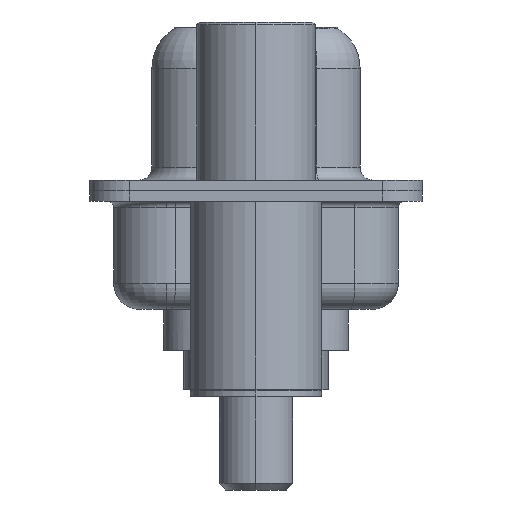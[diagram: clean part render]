
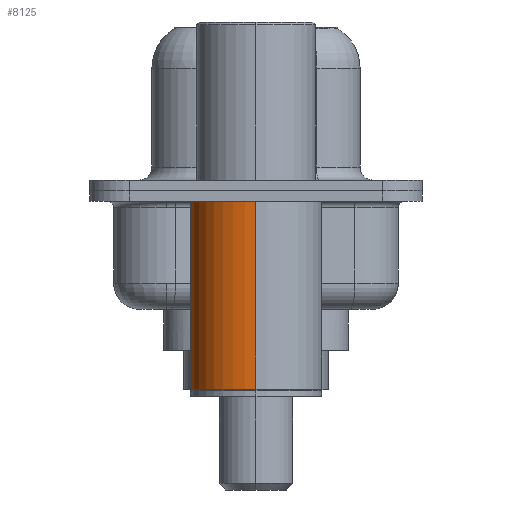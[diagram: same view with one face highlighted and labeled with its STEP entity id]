
A CAD part, left-side view. The second image highlights one B-rep face of the part: STEP entity #8125.
In plain terms, the highlighted cylindrical face has radius 2.5 mm (diameter 5 mm), a partial arc.
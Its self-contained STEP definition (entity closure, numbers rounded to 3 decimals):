
#29 = CARTESIAN_POINT ( 'NONE',  ( 0., 0., 0.581 ) ) ;
#74 = DIRECTION ( 'NONE',  ( 0., 0., 1. ) ) ;
#80 = EDGE_CURVE ( 'NONE', #8897, #9252, #7925, .T. ) ;
#125 = EDGE_CURVE ( 'NONE', #2824, #10675, #13062, .T. ) ;
#345 = AXIS2_PLACEMENT_3D ( 'NONE', #9964, #3302, #11015 ) ;
#373 = AXIS2_PLACEMENT_3D ( 'NONE', #29, #13248, #4343 ) ;
#1049 = VECTOR ( 'NONE', #74, 1000. ) ;
#1395 = CARTESIAN_POINT ( 'NONE',  ( 2.5, 0., 0.581 ) ) ;
#1983 = CARTESIAN_POINT ( 'NONE',  ( 2.5, 0., -0.4 ) ) ;
#2498 = CYLINDRICAL_SURFACE ( 'NONE', #373, 2.5 ) ;
#2824 = VERTEX_POINT ( 'NONE', #4159 ) ;
#3302 = DIRECTION ( 'NONE',  ( 0., 0., 1. ) ) ;
#4159 = CARTESIAN_POINT ( 'NONE',  ( -2.5, 0., -7.525 ) ) ;
#4343 = DIRECTION ( 'NONE',  ( 1., 0., 0. ) ) ;
#4545 = VECTOR ( 'NONE', #8773, 1000. ) ;
#6221 = CARTESIAN_POINT ( 'NONE',  ( 0., 0., -0.4 ) ) ;
#6236 = EDGE_CURVE ( 'NONE', #8897, #2824, #7106, .T. ) ;
#7106 = CIRCLE ( 'NONE', #345, 2.5 ) ;
#7146 = ORIENTED_EDGE ( 'NONE', *, *, #6236, .T. ) ;
#7369 = DIRECTION ( 'NONE',  ( 1., 0., 0. ) ) ;
#7557 = EDGE_CURVE ( 'NONE', #9252, #10675, #11741, .T. ) ;
#7925 = LINE ( 'NONE', #1395, #4545 ) ;
#8109 = ORIENTED_EDGE ( 'NONE', *, *, #80, .F. ) ;
#8125 = ADVANCED_FACE ( 'NONE', ( #8367 ), #2498, .T. ) ;
#8367 = FACE_OUTER_BOUND ( 'NONE', #11936, .T. ) ;
#8773 = DIRECTION ( 'NONE',  ( 0., 0., 1. ) ) ;
#8778 = ORIENTED_EDGE ( 'NONE', *, *, #7557, .F. ) ;
#8897 = VERTEX_POINT ( 'NONE', #11391 ) ;
#9252 = VERTEX_POINT ( 'NONE', #1983 ) ;
#9964 = CARTESIAN_POINT ( 'NONE',  ( 0., 0., -7.525 ) ) ;
#9984 = CARTESIAN_POINT ( 'NONE',  ( -2.5, 0., 0.581 ) ) ;
#10675 = VERTEX_POINT ( 'NONE', #14185 ) ;
#11015 = DIRECTION ( 'NONE',  ( 1., 0., 0. ) ) ;
#11391 = CARTESIAN_POINT ( 'NONE',  ( 2.5, 0., -7.525 ) ) ;
#11741 = CIRCLE ( 'NONE', #12766, 2.5 ) ;
#11936 = EDGE_LOOP ( 'NONE', ( #7146, #14314, #8778, #8109 ) ) ;
#12766 = AXIS2_PLACEMENT_3D ( 'NONE', #6221, #14216, #7369 ) ;
#13062 = LINE ( 'NONE', #9984, #1049 ) ;
#13248 = DIRECTION ( 'NONE',  ( 0., 0., 1. ) ) ;
#14185 = CARTESIAN_POINT ( 'NONE',  ( -2.5, 0., -0.4 ) ) ;
#14216 = DIRECTION ( 'NONE',  ( 0., 0., 1. ) ) ;
#14314 = ORIENTED_EDGE ( 'NONE', *, *, #125, .T. ) ;
